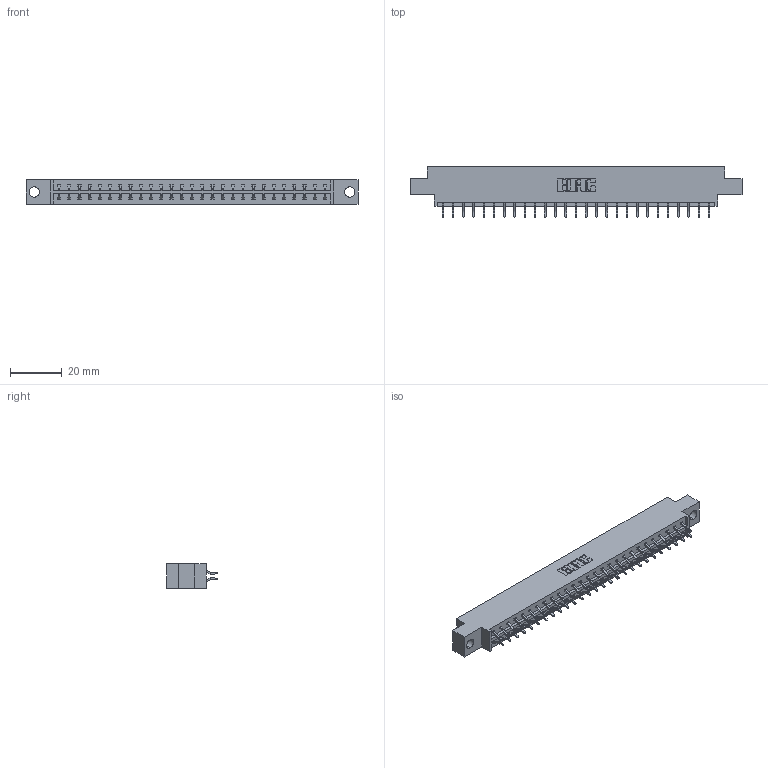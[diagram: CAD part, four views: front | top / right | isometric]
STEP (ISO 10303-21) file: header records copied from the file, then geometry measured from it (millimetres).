
FILE_DESCRIPTION (( 'STEP AP203' ), '1' );
FILE_NAME ('333-054-556-804.STEP', '2018-08-04T04:10:44', ( '' ), ( '' ), 'SwSTEP 2.0', 'SolidWorks 2016', '' );
FILE_SCHEMA (( 'CONFIG_CONTROL_DESIGN' ));
Length unit declared in the file: inch
Products named in the file (3): 333 Part_Offset - .156 Dia - TH; 345-292-001_556 Tail; 333-054-556-804
Assembly tree (55 placements, depth 2):
  333-054-556-804
    333 Part_Offset - .156 Dia - TH
    345-292-001_556 Tail  x54
Bounding box: 128.52 x 19.57 x 9.4 mm (x, y, z)
Volume: 12663.5 mm3; surface area: 14777.2 mm2
Topology: 55 solids, 55 shells, 3250 faces, 9665 edges, 6370 vertices
Faces by surface type: plane 2234, cylinder 1016
Entity records: 19665 total; most frequent: CARTESIAN_POINT 3294, ORIENTED_EDGE 3218, DIRECTION 2829, EDGE_CURVE 1609, LINE 1473, VECTOR 1473, VERTEX_POINT 1070, AXIS2_PLACEMENT_3D 678
